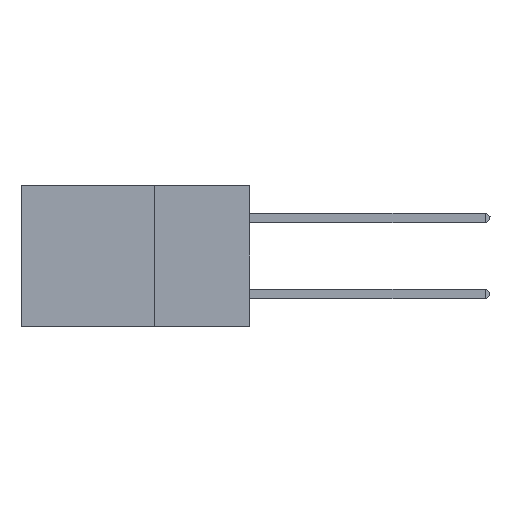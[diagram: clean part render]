
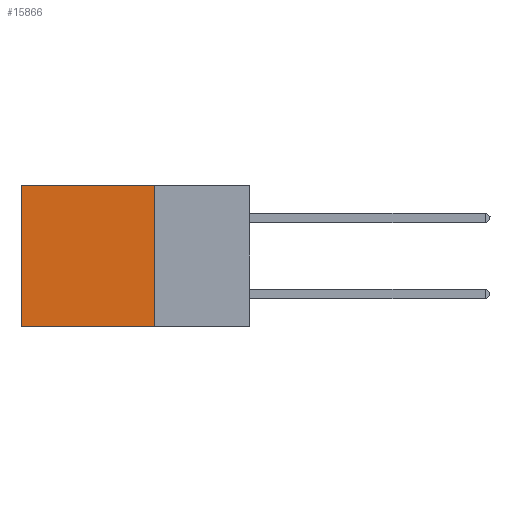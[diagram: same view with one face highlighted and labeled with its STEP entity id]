
A CAD part, left-side view. The second image highlights one B-rep face of the part: STEP entity #15866.
In plain terms, the highlighted planar face has unit normal (-1, 0, 0).
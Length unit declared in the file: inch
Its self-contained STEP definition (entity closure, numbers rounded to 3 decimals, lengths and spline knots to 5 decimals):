
#1166 = VERTEX_POINT ( 'NONE', #16058 ) ;
#1526 = ORIENTED_EDGE ( 'NONE', *, *, #16513, .T. ) ;
#2145 = DIRECTION ( 'NONE',  ( 1., 0., 0. ) ) ;
#3888 = DIRECTION ( 'NONE',  ( 0., 1., 0. ) ) ;
#3944 = EDGE_CURVE ( 'NONE', #7657, #1166, #11313, .T. ) ;
#4424 = VECTOR ( 'NONE', #5448, 39.37008 ) ;
#4722 = DIRECTION ( 'NONE',  ( 0., 0., -1. ) ) ;
#4942 = PLANE ( 'NONE',  #9889 ) ;
#5118 = DIRECTION ( 'NONE',  ( 0., 0., -1. ) ) ;
#5448 = DIRECTION ( 'NONE',  ( 0., 1., 0. ) ) ;
#5721 = CARTESIAN_POINT ( 'NONE',  ( 0.2875, 0.25, -0.37 ) ) ;
#5798 = LINE ( 'NONE', #5887, #7826 ) ;
#5883 = DIRECTION ( 'NONE',  ( 0., 0., -1. ) ) ;
#5887 = CARTESIAN_POINT ( 'NONE',  ( 0.2875, 0.25, 0. ) ) ;
#6119 = LINE ( 'NONE', #7607, #15863 ) ;
#6520 = CARTESIAN_POINT ( 'NONE',  ( 0.2875, 0.25, 0. ) ) ;
#6865 = ORIENTED_EDGE ( 'NONE', *, *, #15316, .T. ) ;
#6985 = VERTEX_POINT ( 'NONE', #7239 ) ;
#7176 = EDGE_CURVE ( 'NONE', #16049, #7657, #6119, .T. ) ;
#7239 = CARTESIAN_POINT ( 'NONE',  ( 0.2875, 0.6, 0. ) ) ;
#7523 = ORIENTED_EDGE ( 'NONE', *, *, #7176, .F. ) ;
#7607 = CARTESIAN_POINT ( 'NONE',  ( 0.2875, 0.25, 0. ) ) ;
#7657 = VERTEX_POINT ( 'NONE', #16472 ) ;
#7826 = VECTOR ( 'NONE', #3888, 39.37008 ) ;
#9071 = LINE ( 'NONE', #16161, #14356 ) ;
#9494 = FACE_OUTER_BOUND ( 'NONE', #15711, .T. ) ;
#9889 = AXIS2_PLACEMENT_3D ( 'NONE', #6520, #2145, #5118 ) ;
#9960 = CARTESIAN_POINT ( 'NONE',  ( 0.2875, 0.25, 0. ) ) ;
#11313 = LINE ( 'NONE', #5721, #4424 ) ;
#14356 = VECTOR ( 'NONE', #5883, 39.37008 ) ;
#14739 = ORIENTED_EDGE ( 'NONE', *, *, #3944, .F. ) ;
#15316 = EDGE_CURVE ( 'NONE', #6985, #1166, #9071, .T. ) ;
#15711 = EDGE_LOOP ( 'NONE', ( #6865, #14739, #7523, #1526 ) ) ;
#15863 = VECTOR ( 'NONE', #4722, 39.37008 ) ;
#15866 = ADVANCED_FACE ( 'NONE', ( #9494 ), #4942, .F. ) ;
#16049 = VERTEX_POINT ( 'NONE', #9960 ) ;
#16058 = CARTESIAN_POINT ( 'NONE',  ( 0.2875, 0.6, -0.37 ) ) ;
#16161 = CARTESIAN_POINT ( 'NONE',  ( 0.2875, 0.6, 0. ) ) ;
#16472 = CARTESIAN_POINT ( 'NONE',  ( 0.2875, 0.25, -0.37 ) ) ;
#16513 = EDGE_CURVE ( 'NONE', #16049, #6985, #5798, .T. ) ;
